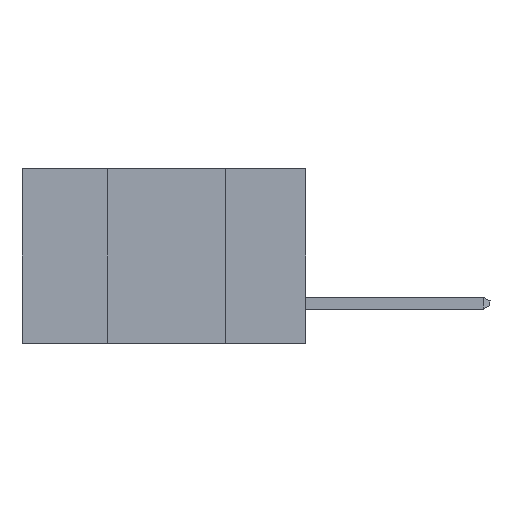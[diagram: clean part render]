
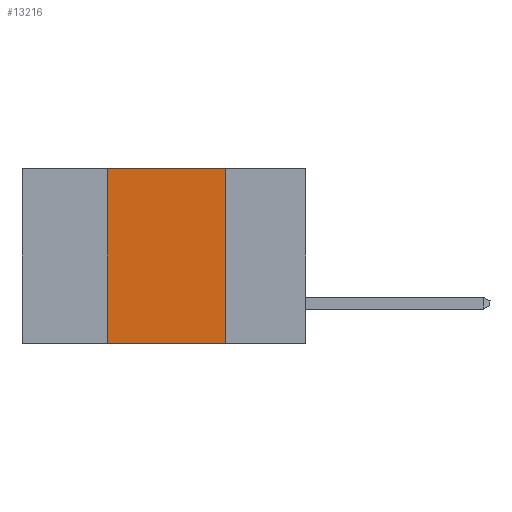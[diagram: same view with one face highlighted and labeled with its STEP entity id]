
A CAD part, left-side view. The second image highlights one B-rep face of the part: STEP entity #13216.
In plain terms, the highlighted planar face has unit normal (-1, 0, 0).
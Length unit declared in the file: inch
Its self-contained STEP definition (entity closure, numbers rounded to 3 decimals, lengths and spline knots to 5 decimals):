
#208 = CARTESIAN_POINT ( 'NONE',  ( 0., 0.6, -0.37 ) ) ;
#647 = DIRECTION ( 'NONE',  ( 0., -1., 0. ) ) ;
#809 = CARTESIAN_POINT ( 'NONE',  ( 0., 0.42, 0. ) ) ;
#2314 = LINE ( 'NONE', #15912, #7603 ) ;
#2457 = VECTOR ( 'NONE', #9914, 39.37008 ) ;
#2925 = EDGE_CURVE ( 'NONE', #15101, #10975, #17017, .T. ) ;
#3091 = CARTESIAN_POINT ( 'NONE',  ( 0., 0.42, -0.37 ) ) ;
#3399 = VECTOR ( 'NONE', #16704, 39.37008 ) ;
#4269 = EDGE_LOOP ( 'NONE', ( #18517, #21161, #18854, #16393 ) ) ;
#5113 = FACE_OUTER_BOUND ( 'NONE', #4269, .T. ) ;
#5351 = CARTESIAN_POINT ( 'NONE',  ( 0., 0.42, -0.37 ) ) ;
#6357 = CARTESIAN_POINT ( 'NONE',  ( 0., 0.17, -0.37 ) ) ;
#7603 = VECTOR ( 'NONE', #647, 39.37008 ) ;
#7913 = CARTESIAN_POINT ( 'NONE',  ( 0., 0.17, 0. ) ) ;
#8464 = DIRECTION ( 'NONE',  ( 0., 0., -1. ) ) ;
#9447 = VERTEX_POINT ( 'NONE', #7913 ) ;
#9736 = EDGE_CURVE ( 'NONE', #19121, #9447, #2314, .T. ) ;
#9914 = DIRECTION ( 'NONE',  ( 0., -1., 0. ) ) ;
#10975 = VERTEX_POINT ( 'NONE', #13832 ) ;
#11478 = LINE ( 'NONE', #6357, #3399 ) ;
#13216 = ADVANCED_FACE ( 'NONE', ( #5113 ), #16902, .F. ) ;
#13832 = CARTESIAN_POINT ( 'NONE',  ( 0., 0.17, -0.37 ) ) ;
#15101 = VERTEX_POINT ( 'NONE', #5351 ) ;
#15765 = VECTOR ( 'NONE', #17109, 39.37008 ) ;
#15912 = CARTESIAN_POINT ( 'NONE',  ( 0., 0.6, 0. ) ) ;
#16393 = ORIENTED_EDGE ( 'NONE', *, *, #2925, .T. ) ;
#16704 = DIRECTION ( 'NONE',  ( 0., 0., -1. ) ) ;
#16788 = DIRECTION ( 'NONE',  ( 1., 0., 0. ) ) ;
#16902 = PLANE ( 'NONE',  #18000 ) ;
#17017 = LINE ( 'NONE', #208, #2457 ) ;
#17051 = EDGE_CURVE ( 'NONE', #15101, #19121, #20428, .T. ) ;
#17109 = DIRECTION ( 'NONE',  ( 0., 0., 1. ) ) ;
#18000 = AXIS2_PLACEMENT_3D ( 'NONE', #18672, #16788, #8464 ) ;
#18517 = ORIENTED_EDGE ( 'NONE', *, *, #21434, .F. ) ;
#18672 = CARTESIAN_POINT ( 'NONE',  ( 0., 0.6, 0. ) ) ;
#18854 = ORIENTED_EDGE ( 'NONE', *, *, #17051, .F. ) ;
#19121 = VERTEX_POINT ( 'NONE', #809 ) ;
#20428 = LINE ( 'NONE', #3091, #15765 ) ;
#21161 = ORIENTED_EDGE ( 'NONE', *, *, #9736, .F. ) ;
#21434 = EDGE_CURVE ( 'NONE', #9447, #10975, #11478, .T. ) ;
